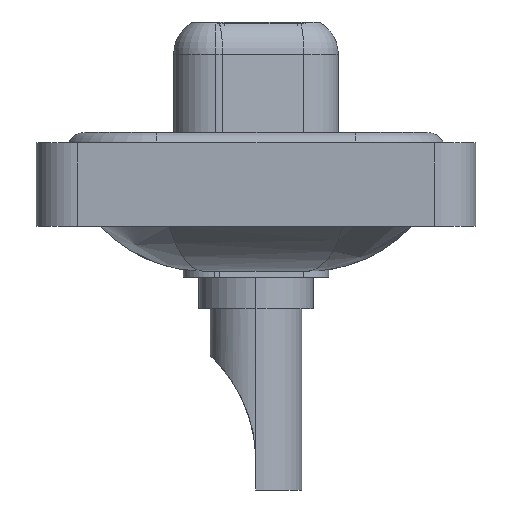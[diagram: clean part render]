
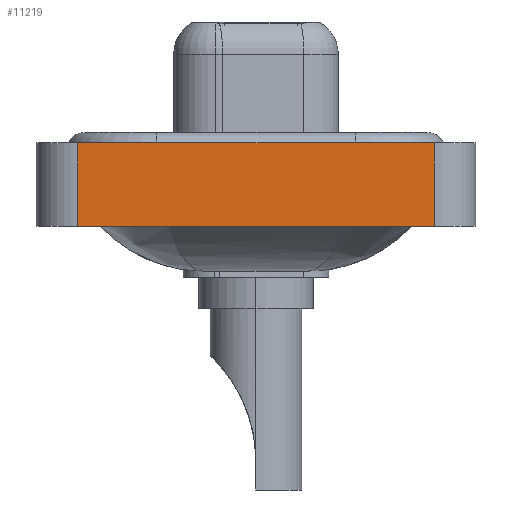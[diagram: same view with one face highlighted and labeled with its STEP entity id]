
A CAD part, left-side view. The second image highlights one B-rep face of the part: STEP entity #11219.
In plain terms, the highlighted planar face has unit normal (-1, 0, 0).
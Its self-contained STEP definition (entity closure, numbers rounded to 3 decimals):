
#482 = EDGE_LOOP ( 'NONE', ( #7209, #9602, #859, #4708 ) ) ;
#859 = ORIENTED_EDGE ( 'NONE', *, *, #2416, .F. ) ;
#1042 = DIRECTION ( 'NONE',  ( 0., 0., 1. ) ) ;
#1383 = DIRECTION ( 'NONE',  ( 0., -1., 0. ) ) ;
#1599 = CARTESIAN_POINT ( 'NONE',  ( -7.3, -8.55, 0.4 ) ) ;
#2296 = LINE ( 'NONE', #12738, #13353 ) ;
#2416 = EDGE_CURVE ( 'NONE', #8668, #10603, #5737, .T. ) ;
#2533 = AXIS2_PLACEMENT_3D ( 'NONE', #10464, #5503, #11706 ) ;
#4428 = FACE_OUTER_BOUND ( 'NONE', #482, .T. ) ;
#4708 = ORIENTED_EDGE ( 'NONE', *, *, #5770, .T. ) ;
#4783 = CARTESIAN_POINT ( 'NONE',  ( -7.3, -8.55, -3.6 ) ) ;
#5418 = CARTESIAN_POINT ( 'NONE',  ( -7.3, 8.55, -3.6 ) ) ;
#5433 = CARTESIAN_POINT ( 'NONE',  ( -7.3, -8.55, -3.6 ) ) ;
#5503 = DIRECTION ( 'NONE',  ( -1., 0., 0. ) ) ;
#5737 = LINE ( 'NONE', #10784, #7202 ) ;
#5770 = EDGE_CURVE ( 'NONE', #8668, #6311, #2296, .T. ) ;
#6123 = CARTESIAN_POINT ( 'NONE',  ( -7.3, 8.55, 0.4 ) ) ;
#6256 = LINE ( 'NONE', #6343, #6607 ) ;
#6311 = VERTEX_POINT ( 'NONE', #5433 ) ;
#6343 = CARTESIAN_POINT ( 'NONE',  ( -7.3, -8.55, 0.4 ) ) ;
#6607 = VECTOR ( 'NONE', #9910, 1000. ) ;
#6819 = DIRECTION ( 'NONE',  ( 0., 0., 1. ) ) ;
#7202 = VECTOR ( 'NONE', #6819, 1000. ) ;
#7209 = ORIENTED_EDGE ( 'NONE', *, *, #15865, .T. ) ;
#8150 = PLANE ( 'NONE',  #2533 ) ;
#8591 = LINE ( 'NONE', #4783, #14875 ) ;
#8668 = VERTEX_POINT ( 'NONE', #5418 ) ;
#9602 = ORIENTED_EDGE ( 'NONE', *, *, #12163, .F. ) ;
#9910 = DIRECTION ( 'NONE',  ( 0., -1., 0. ) ) ;
#10464 = CARTESIAN_POINT ( 'NONE',  ( -7.3, -8.55, -3.6 ) ) ;
#10603 = VERTEX_POINT ( 'NONE', #6123 ) ;
#10784 = CARTESIAN_POINT ( 'NONE',  ( -7.3, 8.55, -3.6 ) ) ;
#11219 = ADVANCED_FACE ( 'NONE', ( #4428 ), #8150, .T. ) ;
#11706 = DIRECTION ( 'NONE',  ( 0., 0., 1. ) ) ;
#12163 = EDGE_CURVE ( 'NONE', #10603, #14393, #6256, .T. ) ;
#12738 = CARTESIAN_POINT ( 'NONE',  ( -7.3, -8.55, -3.6 ) ) ;
#13353 = VECTOR ( 'NONE', #1383, 1000. ) ;
#14393 = VERTEX_POINT ( 'NONE', #1599 ) ;
#14875 = VECTOR ( 'NONE', #1042, 1000. ) ;
#15865 = EDGE_CURVE ( 'NONE', #6311, #14393, #8591, .T. ) ;
